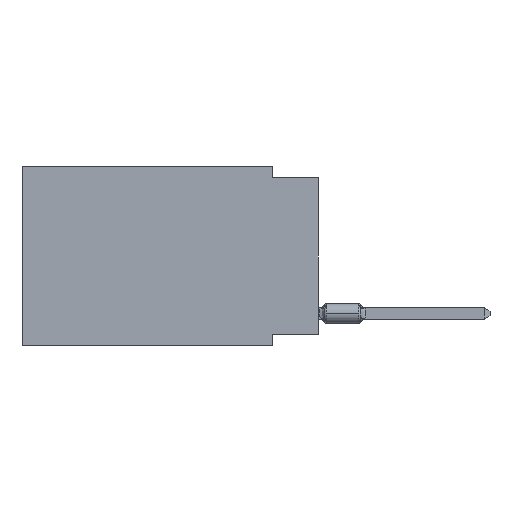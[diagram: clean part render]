
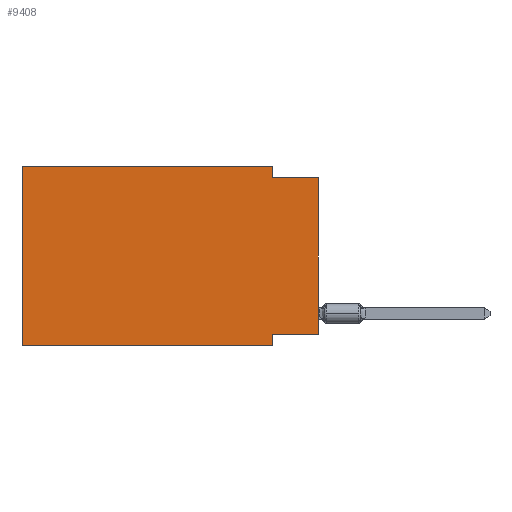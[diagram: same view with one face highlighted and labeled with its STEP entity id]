
A CAD part, left-side view. The second image highlights one B-rep face of the part: STEP entity #9408.
In plain terms, the highlighted planar face has unit normal (-1, 0, 0).
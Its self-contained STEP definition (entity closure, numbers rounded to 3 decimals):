
#426 = DIRECTION ( 'NONE',  ( 0., 0., 1. ) ) ;
#602 = EDGE_CURVE ( 'NONE', #15176, #2386, #8112, .T. ) ;
#764 = FACE_OUTER_BOUND ( 'NONE', #9921, .T. ) ;
#916 = ORIENTED_EDGE ( 'NONE', *, *, #20540, .T. ) ;
#2171 = VECTOR ( 'NONE', #10022, 1000. ) ;
#2299 = EDGE_CURVE ( 'NONE', #11870, #13086, #14232, .T. ) ;
#2386 = VERTEX_POINT ( 'NONE', #17962 ) ;
#2450 = ORIENTED_EDGE ( 'NONE', *, *, #5072, .F. ) ;
#3110 = CARTESIAN_POINT ( 'NONE',  ( 0., 16.383, -9.906 ) ) ;
#3197 = CARTESIAN_POINT ( 'NONE',  ( 0., 0., -9.271 ) ) ;
#3203 = VECTOR ( 'NONE', #16199, 1000. ) ;
#3774 = VECTOR ( 'NONE', #17120, 1000. ) ;
#4256 = EDGE_CURVE ( 'NONE', #6715, #17533, #16851, .T. ) ;
#5072 = EDGE_CURVE ( 'NONE', #2386, #17533, #9122, .T. ) ;
#5366 = CARTESIAN_POINT ( 'NONE',  ( 0., 0., -0.635 ) ) ;
#6468 = CARTESIAN_POINT ( 'NONE',  ( 0., 2.54, -9.271 ) ) ;
#6528 = CARTESIAN_POINT ( 'NONE',  ( 0., 0., 0. ) ) ;
#6715 = VERTEX_POINT ( 'NONE', #3197 ) ;
#7026 = LINE ( 'NONE', #19896, #13437 ) ;
#7033 = ORIENTED_EDGE ( 'NONE', *, *, #7642, .F. ) ;
#7642 = EDGE_CURVE ( 'NONE', #19220, #8084, #13497, .T. ) ;
#8084 = VERTEX_POINT ( 'NONE', #20276 ) ;
#8112 = LINE ( 'NONE', #17798, #2171 ) ;
#8580 = DIRECTION ( 'NONE',  ( 0., 1., 0. ) ) ;
#9122 = LINE ( 'NONE', #10603, #3774 ) ;
#9408 = ADVANCED_FACE ( 'NONE', ( #764 ), #13923, .F. ) ;
#9921 = EDGE_LOOP ( 'NONE', ( #18471, #2450, #17874, #19838, #7033, #916, #20133, #11452 ) ) ;
#10022 = DIRECTION ( 'NONE',  ( 0., 0., -1. ) ) ;
#10603 = CARTESIAN_POINT ( 'NONE',  ( 0., 0., -0.635 ) ) ;
#10622 = DIRECTION ( 'NONE',  ( 1., 0., 0. ) ) ;
#10660 = VECTOR ( 'NONE', #8580, 1000. ) ;
#11452 = ORIENTED_EDGE ( 'NONE', *, *, #14272, .F. ) ;
#11694 = DIRECTION ( 'NONE',  ( 0., -1., 0. ) ) ;
#11785 = CARTESIAN_POINT ( 'NONE',  ( 0., 0., -9.271 ) ) ;
#11870 = VERTEX_POINT ( 'NONE', #6468 ) ;
#12314 = CARTESIAN_POINT ( 'NONE',  ( 0., 2.54, -9.906 ) ) ;
#12580 = EDGE_CURVE ( 'NONE', #8084, #15176, #7026, .T. ) ;
#12782 = LINE ( 'NONE', #3110, #3203 ) ;
#13086 = VERTEX_POINT ( 'NONE', #13364 ) ;
#13136 = DIRECTION ( 'NONE',  ( 0., 0., 1. ) ) ;
#13261 = LINE ( 'NONE', #11785, #10660 ) ;
#13364 = CARTESIAN_POINT ( 'NONE',  ( 0., 2.54, -9.906 ) ) ;
#13437 = VECTOR ( 'NONE', #11694, 1000. ) ;
#13497 = LINE ( 'NONE', #17010, #15785 ) ;
#13923 = PLANE ( 'NONE',  #20243 ) ;
#14056 = VECTOR ( 'NONE', #15528, 1000. ) ;
#14148 = VECTOR ( 'NONE', #13136, 1000. ) ;
#14232 = LINE ( 'NONE', #12314, #14056 ) ;
#14272 = EDGE_CURVE ( 'NONE', #6715, #11870, #13261, .T. ) ;
#15176 = VERTEX_POINT ( 'NONE', #16852 ) ;
#15528 = DIRECTION ( 'NONE',  ( 0., 0., -1. ) ) ;
#15745 = CARTESIAN_POINT ( 'NONE',  ( 0., 16.383, 0. ) ) ;
#15785 = VECTOR ( 'NONE', #426, 1000. ) ;
#16199 = DIRECTION ( 'NONE',  ( 0., -1., 0. ) ) ;
#16851 = LINE ( 'NONE', #6528, #14148 ) ;
#16852 = CARTESIAN_POINT ( 'NONE',  ( 0., 2.54, 0. ) ) ;
#17010 = CARTESIAN_POINT ( 'NONE',  ( 0., 16.383, 0. ) ) ;
#17048 = CARTESIAN_POINT ( 'NONE',  ( 0., 16.383, -9.906 ) ) ;
#17120 = DIRECTION ( 'NONE',  ( 0., -1., 0. ) ) ;
#17145 = DIRECTION ( 'NONE',  ( 0., 0., -1. ) ) ;
#17533 = VERTEX_POINT ( 'NONE', #5366 ) ;
#17798 = CARTESIAN_POINT ( 'NONE',  ( 0., 2.54, 0. ) ) ;
#17874 = ORIENTED_EDGE ( 'NONE', *, *, #602, .F. ) ;
#17962 = CARTESIAN_POINT ( 'NONE',  ( 0., 2.54, -0.635 ) ) ;
#18471 = ORIENTED_EDGE ( 'NONE', *, *, #4256, .T. ) ;
#19220 = VERTEX_POINT ( 'NONE', #17048 ) ;
#19838 = ORIENTED_EDGE ( 'NONE', *, *, #12580, .F. ) ;
#19896 = CARTESIAN_POINT ( 'NONE',  ( 0., 16.383, 0. ) ) ;
#20133 = ORIENTED_EDGE ( 'NONE', *, *, #2299, .F. ) ;
#20243 = AXIS2_PLACEMENT_3D ( 'NONE', #15745, #10622, #17145 ) ;
#20276 = CARTESIAN_POINT ( 'NONE',  ( 0., 16.383, 0. ) ) ;
#20540 = EDGE_CURVE ( 'NONE', #19220, #13086, #12782, .T. ) ;
